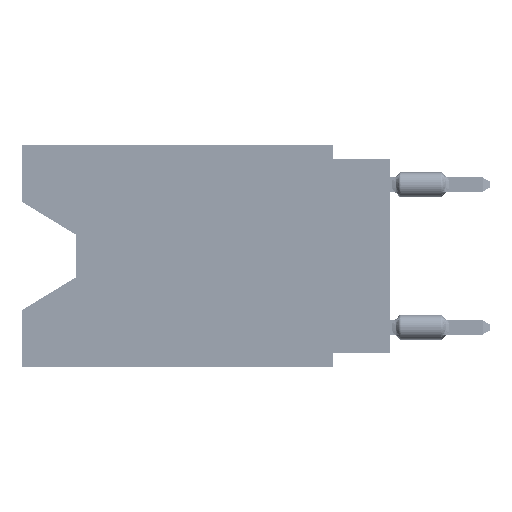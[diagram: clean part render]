
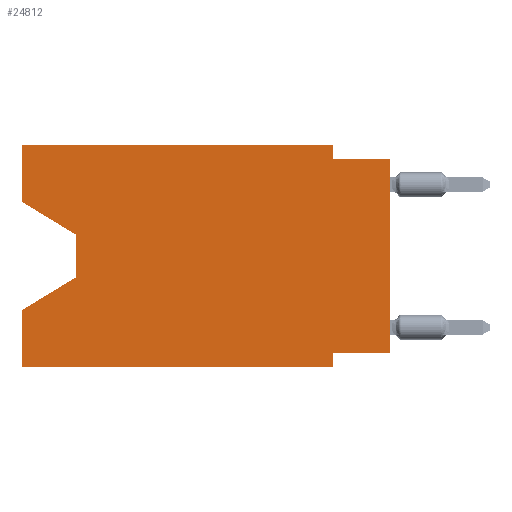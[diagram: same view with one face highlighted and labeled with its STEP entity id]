
A CAD part, left-side view. The second image highlights one B-rep face of the part: STEP entity #24812.
In plain terms, the highlighted planar face has unit normal (-1, 0, 0).
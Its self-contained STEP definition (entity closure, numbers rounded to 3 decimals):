
#1066 = CARTESIAN_POINT ( 'NONE',  ( 0., 16.383, 0. ) ) ;
#1112 = VERTEX_POINT ( 'NONE', #10886 ) ;
#1127 = VERTEX_POINT ( 'NONE', #1066 ) ;
#2010 = CARTESIAN_POINT ( 'NONE',  ( 0., 16.383, -7.36 ) ) ;
#2248 = ORIENTED_EDGE ( 'NONE', *, *, #40377, .T. ) ;
#3254 = ORIENTED_EDGE ( 'NONE', *, *, #51615, .T. ) ;
#4099 = DIRECTION ( 'NONE',  ( 0., 0., 1. ) ) ;
#4663 = CARTESIAN_POINT ( 'NONE',  ( 0., 16.383, 0. ) ) ;
#4700 = ORIENTED_EDGE ( 'NONE', *, *, #55674, .T. ) ;
#4727 = ORIENTED_EDGE ( 'NONE', *, *, #18999, .F. ) ;
#5522 = VERTEX_POINT ( 'NONE', #17476 ) ;
#5784 = CARTESIAN_POINT ( 'NONE',  ( 0., 2.54, 0. ) ) ;
#5853 = DIRECTION ( 'NONE',  ( 0., 0., 1. ) ) ;
#6580 = VECTOR ( 'NONE', #25154, 1000. ) ;
#7939 = CARTESIAN_POINT ( 'NONE',  ( 0., 13.97, -5.893 ) ) ;
#8579 = CARTESIAN_POINT ( 'NONE',  ( 0., 2.54, 0. ) ) ;
#8656 = VECTOR ( 'NONE', #41360, 1000. ) ;
#9440 = LINE ( 'NONE', #35305, #6580 ) ;
#9738 = CARTESIAN_POINT ( 'NONE',  ( 0., 13.97, -4.013 ) ) ;
#10827 = EDGE_LOOP ( 'NONE', ( #35524, #2248, #64857, #40851, #3254, #43740, #4727, #4700, #45791, #68407, #50893, #38351 ) ) ;
#10886 = CARTESIAN_POINT ( 'NONE',  ( 0., 13.97, -4.013 ) ) ;
#11162 = CARTESIAN_POINT ( 'NONE',  ( 0., 0., -0.635 ) ) ;
#11170 = CARTESIAN_POINT ( 'NONE',  ( 0., 16.383, 0. ) ) ;
#11254 = CARTESIAN_POINT ( 'NONE',  ( 0., 2.54, -9.906 ) ) ;
#12822 = CARTESIAN_POINT ( 'NONE',  ( 0., 2.54, -0.635 ) ) ;
#13787 = EDGE_CURVE ( 'NONE', #1127, #51435, #21100, .T. ) ;
#16237 = CARTESIAN_POINT ( 'NONE',  ( 0., 16.383, -2.546 ) ) ;
#16672 = CARTESIAN_POINT ( 'NONE',  ( 0., 2.54, -9.906 ) ) ;
#16953 = VECTOR ( 'NONE', #42860, 1000. ) ;
#17476 = CARTESIAN_POINT ( 'NONE',  ( 0., 2.54, -9.271 ) ) ;
#18651 = VECTOR ( 'NONE', #39905, 1000. ) ;
#18997 = AXIS2_PLACEMENT_3D ( 'NONE', #11170, #22323, #27563 ) ;
#18999 = EDGE_CURVE ( 'NONE', #30811, #5522, #63125, .T. ) ;
#19524 = LINE ( 'NONE', #9738, #68759 ) ;
#21100 = LINE ( 'NONE', #4663, #8656 ) ;
#22323 = DIRECTION ( 'NONE',  ( 1., 0., 0. ) ) ;
#24812 = ADVANCED_FACE ( 'NONE', ( #26175 ), #37019, .F. ) ;
#25154 = DIRECTION ( 'NONE',  ( 0., 0.855, -0.519 ) ) ;
#25232 = DIRECTION ( 'NONE',  ( 0., -0.855, -0.519 ) ) ;
#25406 = CARTESIAN_POINT ( 'NONE',  ( 0., 16.383, 0. ) ) ;
#26168 = LINE ( 'NONE', #11162, #43029 ) ;
#26175 = FACE_OUTER_BOUND ( 'NONE', #10827, .T. ) ;
#26372 = VECTOR ( 'NONE', #25232, 1000. ) ;
#27563 = DIRECTION ( 'NONE',  ( 0., 0., -1. ) ) ;
#29341 = VECTOR ( 'NONE', #60182, 1000. ) ;
#29753 = CARTESIAN_POINT ( 'NONE',  ( 0., 16.383, -9.906 ) ) ;
#30307 = LINE ( 'NONE', #25406, #65086 ) ;
#30811 = VERTEX_POINT ( 'NONE', #58541 ) ;
#31342 = CARTESIAN_POINT ( 'NONE',  ( 0., 0., -9.271 ) ) ;
#31491 = CARTESIAN_POINT ( 'NONE',  ( 0., 0., -0.635 ) ) ;
#32395 = LINE ( 'NONE', #16672, #29341 ) ;
#32412 = CARTESIAN_POINT ( 'NONE',  ( 0., 16.383, 0. ) ) ;
#34101 = DIRECTION ( 'NONE',  ( 0., 0., -1. ) ) ;
#35305 = CARTESIAN_POINT ( 'NONE',  ( 0., 13.97, -5.893 ) ) ;
#35524 = ORIENTED_EDGE ( 'NONE', *, *, #68243, .T. ) ;
#35717 = LINE ( 'NONE', #58406, #26372 ) ;
#37019 = PLANE ( 'NONE',  #18997 ) ;
#37652 = DIRECTION ( 'NONE',  ( 0., 0., 1. ) ) ;
#38351 = ORIENTED_EDGE ( 'NONE', *, *, #55671, .F. ) ;
#39905 = DIRECTION ( 'NONE',  ( 0., -1., 0. ) ) ;
#40320 = CARTESIAN_POINT ( 'NONE',  ( 0., 16.383, -9.906 ) ) ;
#40377 = EDGE_CURVE ( 'NONE', #1112, #52447, #19524, .T. ) ;
#40851 = ORIENTED_EDGE ( 'NONE', *, *, #61095, .F. ) ;
#41360 = DIRECTION ( 'NONE',  ( 0., -1., 0. ) ) ;
#42860 = DIRECTION ( 'NONE',  ( 0., 1., 0. ) ) ;
#42887 = LINE ( 'NONE', #32412, #56935 ) ;
#43029 = VECTOR ( 'NONE', #48183, 1000. ) ;
#43613 = EDGE_CURVE ( 'NONE', #52447, #57084, #9440, .T. ) ;
#43740 = ORIENTED_EDGE ( 'NONE', *, *, #51004, .F. ) ;
#45791 = ORIENTED_EDGE ( 'NONE', *, *, #49220, .F. ) ;
#46202 = VERTEX_POINT ( 'NONE', #40320 ) ;
#47624 = VERTEX_POINT ( 'NONE', #31491 ) ;
#48183 = DIRECTION ( 'NONE',  ( 0., -1., 0. ) ) ;
#48625 = VECTOR ( 'NONE', #34101, 1000. ) ;
#49220 = EDGE_CURVE ( 'NONE', #55819, #47624, #26168, .T. ) ;
#50893 = ORIENTED_EDGE ( 'NONE', *, *, #13787, .F. ) ;
#51004 = EDGE_CURVE ( 'NONE', #5522, #63562, #32395, .T. ) ;
#51435 = VERTEX_POINT ( 'NONE', #5784 ) ;
#51615 = EDGE_CURVE ( 'NONE', #46202, #63562, #56997, .T. ) ;
#52447 = VERTEX_POINT ( 'NONE', #7939 ) ;
#53726 = LINE ( 'NONE', #68743, #63657 ) ;
#55671 = EDGE_CURVE ( 'NONE', #69034, #1127, #42887, .T. ) ;
#55674 = EDGE_CURVE ( 'NONE', #30811, #47624, #53726, .T. ) ;
#55819 = VERTEX_POINT ( 'NONE', #12822 ) ;
#56935 = VECTOR ( 'NONE', #37652, 1000. ) ;
#56997 = LINE ( 'NONE', #29753, #18651 ) ;
#57084 = VERTEX_POINT ( 'NONE', #2010 ) ;
#58406 = CARTESIAN_POINT ( 'NONE',  ( 0., 16.383, -2.546 ) ) ;
#58541 = CARTESIAN_POINT ( 'NONE',  ( 0., 0., -9.271 ) ) ;
#60182 = DIRECTION ( 'NONE',  ( 0., 0., -1. ) ) ;
#60653 = LINE ( 'NONE', #8579, #48625 ) ;
#61095 = EDGE_CURVE ( 'NONE', #46202, #57084, #30307, .T. ) ;
#63125 = LINE ( 'NONE', #31342, #16953 ) ;
#63562 = VERTEX_POINT ( 'NONE', #11254 ) ;
#63657 = VECTOR ( 'NONE', #5853, 1000. ) ;
#64147 = EDGE_CURVE ( 'NONE', #51435, #55819, #60653, .T. ) ;
#64857 = ORIENTED_EDGE ( 'NONE', *, *, #43613, .T. ) ;
#65086 = VECTOR ( 'NONE', #4099, 1000. ) ;
#68065 = DIRECTION ( 'NONE',  ( 0., 0., -1. ) ) ;
#68243 = EDGE_CURVE ( 'NONE', #69034, #1112, #35717, .T. ) ;
#68407 = ORIENTED_EDGE ( 'NONE', *, *, #64147, .F. ) ;
#68743 = CARTESIAN_POINT ( 'NONE',  ( 0., 0., 0. ) ) ;
#68759 = VECTOR ( 'NONE', #68065, 1000. ) ;
#69034 = VERTEX_POINT ( 'NONE', #16237 ) ;
